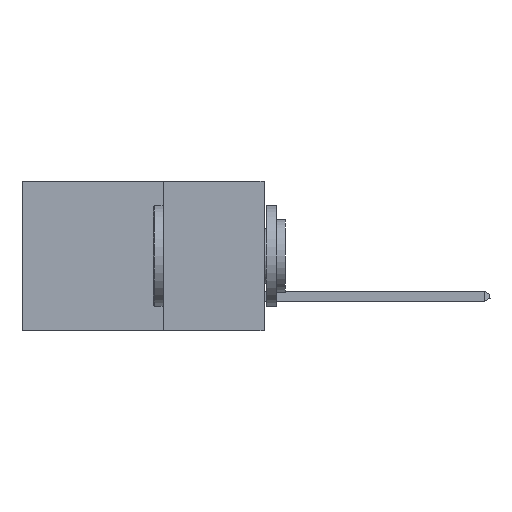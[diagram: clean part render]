
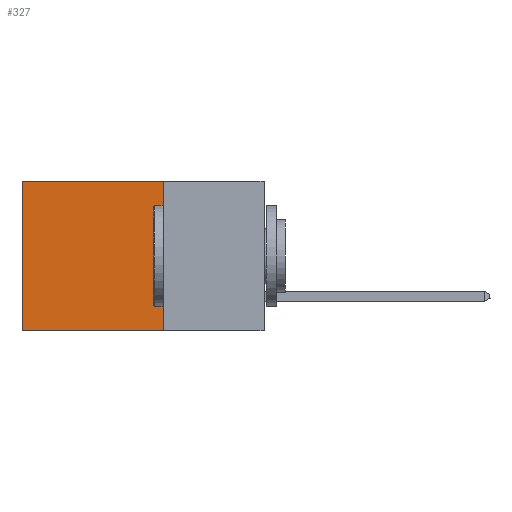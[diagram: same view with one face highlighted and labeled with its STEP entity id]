
A CAD part, left-side view. The second image highlights one B-rep face of the part: STEP entity #327.
In plain terms, the highlighted planar face has unit normal (-1, 0, 0).
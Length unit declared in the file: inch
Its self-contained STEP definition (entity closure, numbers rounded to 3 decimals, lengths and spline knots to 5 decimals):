
#327 = ADVANCED_FACE ( 'NONE', ( #21095 ), #26709, .F. ) ;
#4512 = AXIS2_PLACEMENT_3D ( 'NONE', #28978, #21710, #6948 ) ;
#5137 = DIRECTION ( 'NONE',  ( 0., 1., 0. ) ) ;
#5703 = CARTESIAN_POINT ( 'NONE',  ( 0.298, 0.25, 0. ) ) ;
#6318 = CARTESIAN_POINT ( 'NONE',  ( 0.298, 0.6, -0.37 ) ) ;
#6948 = DIRECTION ( 'NONE',  ( 0., 0., -1. ) ) ;
#7173 = ORIENTED_EDGE ( 'NONE', *, *, #28463, .T. ) ;
#7539 = ORIENTED_EDGE ( 'NONE', *, *, #16722, .F. ) ;
#8623 = VERTEX_POINT ( 'NONE', #16421 ) ;
#9015 = CARTESIAN_POINT ( 'NONE',  ( 0.298, 0.6, 0. ) ) ;
#10350 = VERTEX_POINT ( 'NONE', #6318 ) ;
#11238 = VERTEX_POINT ( 'NONE', #5703 ) ;
#12272 = CARTESIAN_POINT ( 'NONE',  ( 0.298, 0.25, 0. ) ) ;
#13828 = LINE ( 'NONE', #18203, #14922 ) ;
#14373 = EDGE_CURVE ( 'NONE', #28684, #10350, #20079, .T. ) ;
#14702 = CARTESIAN_POINT ( 'NONE',  ( 0.298, 0.6, 0. ) ) ;
#14922 = VECTOR ( 'NONE', #15766, 39.37008 ) ;
#15630 = ORIENTED_EDGE ( 'NONE', *, *, #17512, .F. ) ;
#15766 = DIRECTION ( 'NONE',  ( 0., 1., 0. ) ) ;
#16097 = LINE ( 'NONE', #12272, #19126 ) ;
#16421 = CARTESIAN_POINT ( 'NONE',  ( 0.298, 0.25, -0.37 ) ) ;
#16722 = EDGE_CURVE ( 'NONE', #11238, #8623, #28614, .T. ) ;
#16807 = EDGE_LOOP ( 'NONE', ( #22829, #15630, #7539, #7173 ) ) ;
#17512 = EDGE_CURVE ( 'NONE', #8623, #10350, #13828, .T. ) ;
#18203 = CARTESIAN_POINT ( 'NONE',  ( 0.298, 0.25, -0.37 ) ) ;
#18396 = CARTESIAN_POINT ( 'NONE',  ( 0.298, 0.25, 0. ) ) ;
#19126 = VECTOR ( 'NONE', #5137, 39.37008 ) ;
#19152 = VECTOR ( 'NONE', #23029, 39.37008 ) ;
#20079 = LINE ( 'NONE', #9015, #29517 ) ;
#21095 = FACE_OUTER_BOUND ( 'NONE', #16807, .T. ) ;
#21710 = DIRECTION ( 'NONE',  ( 1., 0., 0. ) ) ;
#22829 = ORIENTED_EDGE ( 'NONE', *, *, #14373, .T. ) ;
#23029 = DIRECTION ( 'NONE',  ( 0., 0., -1. ) ) ;
#26709 = PLANE ( 'NONE',  #4512 ) ;
#28463 = EDGE_CURVE ( 'NONE', #11238, #28684, #16097, .T. ) ;
#28614 = LINE ( 'NONE', #18396, #19152 ) ;
#28684 = VERTEX_POINT ( 'NONE', #14702 ) ;
#28978 = CARTESIAN_POINT ( 'NONE',  ( 0.298, 0.25, 0. ) ) ;
#29517 = VECTOR ( 'NONE', #30826, 39.37008 ) ;
#30826 = DIRECTION ( 'NONE',  ( 0., 0., -1. ) ) ;
